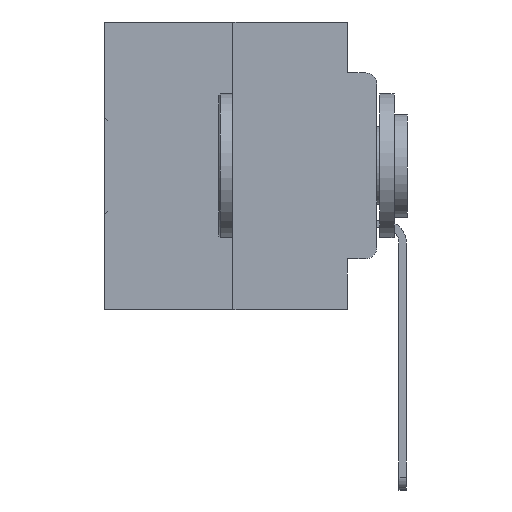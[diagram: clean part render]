
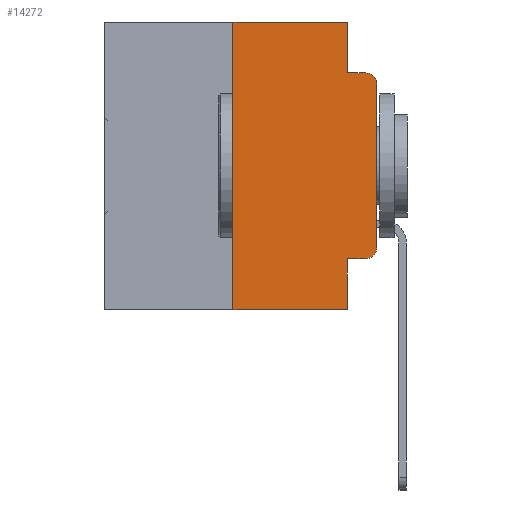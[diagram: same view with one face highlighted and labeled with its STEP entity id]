
A CAD part, left-side view. The second image highlights one B-rep face of the part: STEP entity #14272.
In plain terms, the highlighted planar face has unit normal (-1, 0, 0).
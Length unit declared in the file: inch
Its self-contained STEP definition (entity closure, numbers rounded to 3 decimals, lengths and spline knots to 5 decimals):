
#145 = CARTESIAN_POINT ( 'NONE',  ( 0., 0.473, 0. ) ) ;
#727 = ORIENTED_EDGE ( 'NONE', *, *, #25200, .F. ) ;
#1174 = DIRECTION ( 'NONE',  ( -1., 0., 0. ) ) ;
#1682 = VERTEX_POINT ( 'NONE', #18253 ) ;
#1841 = CARTESIAN_POINT ( 'NONE',  ( 0., 0.051, -0.4115 ) ) ;
#1984 = CARTESIAN_POINT ( 'NONE',  ( 0., 0.051, -0.0885 ) ) ;
#2151 = DIRECTION ( 'NONE',  ( 0., -1., 0. ) ) ;
#3479 = DIRECTION ( 'NONE',  ( 0., 0., 1. ) ) ;
#5051 = CARTESIAN_POINT ( 'NONE',  ( 0., 0.051, -0.5 ) ) ;
#5906 = VERTEX_POINT ( 'NONE', #5051 ) ;
#7297 = CARTESIAN_POINT ( 'NONE',  ( 0., 0.473, -0.5 ) ) ;
#7749 = LINE ( 'NONE', #20158, #20615 ) ;
#8155 = VERTEX_POINT ( 'NONE', #29939 ) ;
#8174 = ORIENTED_EDGE ( 'NONE', *, *, #11385, .F. ) ;
#9424 = VERTEX_POINT ( 'NONE', #18276 ) ;
#9505 = AXIS2_PLACEMENT_3D ( 'NONE', #16803, #1174, #19355 ) ;
#9582 = CARTESIAN_POINT ( 'NONE',  ( 0., 0.02, -0.1085 ) ) ;
#9625 = EDGE_CURVE ( 'NONE', #31751, #26859, #23489, .T. ) ;
#9904 = VECTOR ( 'NONE', #14010, 39.37008 ) ;
#10228 = ORIENTED_EDGE ( 'NONE', *, *, #14143, .T. ) ;
#10426 = CARTESIAN_POINT ( 'NONE',  ( 0., 0., -0.3915 ) ) ;
#11385 = EDGE_CURVE ( 'NONE', #26859, #8155, #7749, .T. ) ;
#11436 = FACE_OUTER_BOUND ( 'NONE', #26429, .T. ) ;
#11514 = VERTEX_POINT ( 'NONE', #33051 ) ;
#12097 = PLANE ( 'NONE',  #28269 ) ;
#12230 = DIRECTION ( 'NONE',  ( 0., 0., -1. ) ) ;
#12469 = VECTOR ( 'NONE', #18399, 39.37008 ) ;
#12484 = EDGE_CURVE ( 'NONE', #30044, #11514, #13780, .T. ) ;
#13780 = LINE ( 'NONE', #26546, #25679 ) ;
#14010 = DIRECTION ( 'NONE',  ( 0., 0., -1. ) ) ;
#14143 = EDGE_CURVE ( 'NONE', #17099, #30044, #28913, .T. ) ;
#14258 = LINE ( 'NONE', #16422, #14615 ) ;
#14272 = ADVANCED_FACE ( 'NONE', ( #11436 ), #12097, .F. ) ;
#14394 = DIRECTION ( 'NONE',  ( 0., 0., -1. ) ) ;
#14615 = VECTOR ( 'NONE', #3479, 39.37008 ) ;
#16310 = CIRCLE ( 'NONE', #27477, 0.02 ) ;
#16422 = CARTESIAN_POINT ( 'NONE',  ( 0., 0.25, 0. ) ) ;
#16803 = CARTESIAN_POINT ( 'NONE',  ( 0., 0.02, -0.3915 ) ) ;
#17099 = VERTEX_POINT ( 'NONE', #28647 ) ;
#17249 = DIRECTION ( 'NONE',  ( 0., 0., -1. ) ) ;
#17463 = DIRECTION ( 'NONE',  ( 0., -1., 0. ) ) ;
#17699 = DIRECTION ( 'NONE',  ( 0., -1., 0. ) ) ;
#17749 = VECTOR ( 'NONE', #17463, 39.37008 ) ;
#18253 = CARTESIAN_POINT ( 'NONE',  ( 0., 0.051, -0.4115 ) ) ;
#18262 = EDGE_CURVE ( 'NONE', #11514, #8155, #16310, .T. ) ;
#18276 = CARTESIAN_POINT ( 'NONE',  ( 0., 0.25, -0.5 ) ) ;
#18362 = EDGE_CURVE ( 'NONE', #9424, #5906, #26552, .T. ) ;
#18399 = DIRECTION ( 'NONE',  ( 0., -1., 0. ) ) ;
#18645 = ORIENTED_EDGE ( 'NONE', *, *, #12484, .T. ) ;
#19255 = LINE ( 'NONE', #145, #12469 ) ;
#19355 = DIRECTION ( 'NONE',  ( 0., 0., -1. ) ) ;
#19864 = VECTOR ( 'NONE', #17699, 39.37008 ) ;
#20158 = CARTESIAN_POINT ( 'NONE',  ( 0., 0.051, -0.0885 ) ) ;
#20615 = VECTOR ( 'NONE', #2151, 39.37008 ) ;
#20633 = ORIENTED_EDGE ( 'NONE', *, *, #18362, .T. ) ;
#21457 = CARTESIAN_POINT ( 'NONE',  ( 0., 0.051, 0. ) ) ;
#23388 = ORIENTED_EDGE ( 'NONE', *, *, #9625, .F. ) ;
#23489 = LINE ( 'NONE', #21457, #9904 ) ;
#23656 = LINE ( 'NONE', #1841, #17749 ) ;
#24555 = LINE ( 'NONE', #29543, #25358 ) ;
#25200 = EDGE_CURVE ( 'NONE', #1682, #5906, #24555, .T. ) ;
#25358 = VECTOR ( 'NONE', #14394, 39.37008 ) ;
#25679 = VECTOR ( 'NONE', #26646, 39.37008 ) ;
#25753 = ORIENTED_EDGE ( 'NONE', *, *, #29671, .F. ) ;
#26127 = ORIENTED_EDGE ( 'NONE', *, *, #18262, .T. ) ;
#26429 = EDGE_LOOP ( 'NONE', ( #18645, #26127, #8174, #23388, #31704, #25753, #20633, #727, #29725, #10228 ) ) ;
#26546 = CARTESIAN_POINT ( 'NONE',  ( 0., 0., 0. ) ) ;
#26552 = LINE ( 'NONE', #7297, #19864 ) ;
#26646 = DIRECTION ( 'NONE',  ( 0., 0., 1. ) ) ;
#26859 = VERTEX_POINT ( 'NONE', #1984 ) ;
#27392 = DIRECTION ( 'NONE',  ( -1., 0., 0. ) ) ;
#27477 = AXIS2_PLACEMENT_3D ( 'NONE', #9582, #27392, #12230 ) ;
#27765 = EDGE_CURVE ( 'NONE', #28174, #31751, #19255, .T. ) ;
#28174 = VERTEX_POINT ( 'NONE', #30105 ) ;
#28269 = AXIS2_PLACEMENT_3D ( 'NONE', #29831, #32395, #17249 ) ;
#28647 = CARTESIAN_POINT ( 'NONE',  ( 0., 0.02, -0.4115 ) ) ;
#28913 = CIRCLE ( 'NONE', #9505, 0.02 ) ;
#29543 = CARTESIAN_POINT ( 'NONE',  ( 0., 0.051, 0. ) ) ;
#29671 = EDGE_CURVE ( 'NONE', #9424, #28174, #14258, .T. ) ;
#29725 = ORIENTED_EDGE ( 'NONE', *, *, #31112, .T. ) ;
#29831 = CARTESIAN_POINT ( 'NONE',  ( 0., 0.473, 0. ) ) ;
#29887 = CARTESIAN_POINT ( 'NONE',  ( 0., 0.051, 0. ) ) ;
#29939 = CARTESIAN_POINT ( 'NONE',  ( 0., 0.02, -0.0885 ) ) ;
#30044 = VERTEX_POINT ( 'NONE', #10426 ) ;
#30105 = CARTESIAN_POINT ( 'NONE',  ( 0., 0.25, 0. ) ) ;
#31112 = EDGE_CURVE ( 'NONE', #1682, #17099, #23656, .T. ) ;
#31704 = ORIENTED_EDGE ( 'NONE', *, *, #27765, .F. ) ;
#31751 = VERTEX_POINT ( 'NONE', #29887 ) ;
#32395 = DIRECTION ( 'NONE',  ( 1., 0., 0. ) ) ;
#33051 = CARTESIAN_POINT ( 'NONE',  ( 0., 0., -0.1085 ) ) ;
